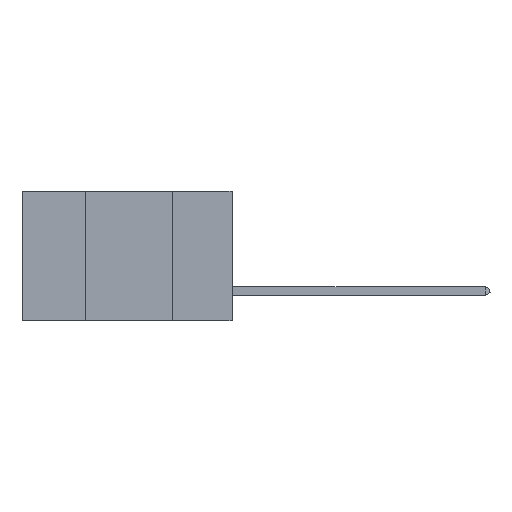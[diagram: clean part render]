
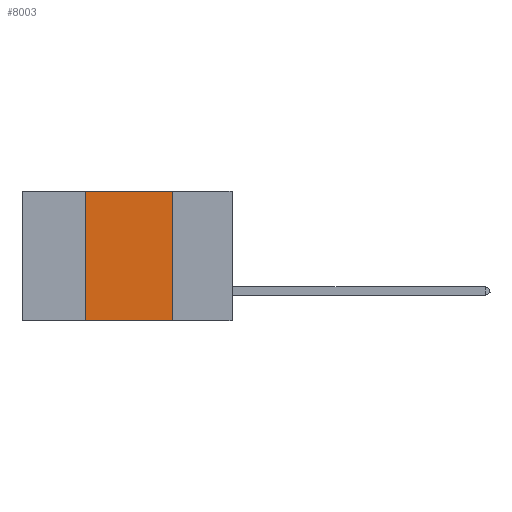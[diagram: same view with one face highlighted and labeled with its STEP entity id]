
A CAD part, left-side view. The second image highlights one B-rep face of the part: STEP entity #8003.
In plain terms, the highlighted planar face has unit normal (-1, 0, 0).
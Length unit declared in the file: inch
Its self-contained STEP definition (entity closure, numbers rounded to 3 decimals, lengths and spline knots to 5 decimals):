
#349 = VERTEX_POINT ( 'NONE', #8921 ) ;
#2960 = CARTESIAN_POINT ( 'NONE',  ( 0., 0.42, 0. ) ) ;
#4209 = VERTEX_POINT ( 'NONE', #22917 ) ;
#7087 = LINE ( 'NONE', #13964, #18270 ) ;
#8003 = ADVANCED_FACE ( 'NONE', ( #25514 ), #35412, .F. ) ;
#8921 = CARTESIAN_POINT ( 'NONE',  ( 0., 0.17, 0. ) ) ;
#9891 = DIRECTION ( 'NONE',  ( 0., -1., 0. ) ) ;
#11871 = VERTEX_POINT ( 'NONE', #13775 ) ;
#12262 = CARTESIAN_POINT ( 'NONE',  ( 0., 0.6, -0.37 ) ) ;
#13615 = VERTEX_POINT ( 'NONE', #2960 ) ;
#13775 = CARTESIAN_POINT ( 'NONE',  ( 0., 0.42, -0.37 ) ) ;
#13964 = CARTESIAN_POINT ( 'NONE',  ( 0., 0.17, 0. ) ) ;
#15202 = DIRECTION ( 'NONE',  ( 1., 0., 0. ) ) ;
#15417 = CARTESIAN_POINT ( 'NONE',  ( 0., 0.6, 0. ) ) ;
#17225 = DIRECTION ( 'NONE',  ( 0., 0., 1. ) ) ;
#18270 = VECTOR ( 'NONE', #40612, 39.37008 ) ;
#18749 = CARTESIAN_POINT ( 'NONE',  ( 0., 0.6, 0. ) ) ;
#19337 = LINE ( 'NONE', #12262, #34757 ) ;
#22237 = EDGE_CURVE ( 'NONE', #11871, #13615, #36586, .T. ) ;
#22614 = EDGE_CURVE ( 'NONE', #349, #4209, #7087, .T. ) ;
#22917 = CARTESIAN_POINT ( 'NONE',  ( 0., 0.17, -0.37 ) ) ;
#23212 = ORIENTED_EDGE ( 'NONE', *, *, #22237, .F. ) ;
#23309 = EDGE_CURVE ( 'NONE', #13615, #349, #34316, .T. ) ;
#25514 = FACE_OUTER_BOUND ( 'NONE', #37423, .T. ) ;
#33944 = AXIS2_PLACEMENT_3D ( 'NONE', #15417, #15202, #38408 ) ;
#34316 = LINE ( 'NONE', #18749, #36861 ) ;
#34451 = ORIENTED_EDGE ( 'NONE', *, *, #23309, .F. ) ;
#34757 = VECTOR ( 'NONE', #9891, 39.37008 ) ;
#35412 = PLANE ( 'NONE',  #33944 ) ;
#35606 = EDGE_CURVE ( 'NONE', #11871, #4209, #19337, .T. ) ;
#36586 = LINE ( 'NONE', #36799, #41613 ) ;
#36799 = CARTESIAN_POINT ( 'NONE',  ( 0., 0.42, 0. ) ) ;
#36861 = VECTOR ( 'NONE', #38534, 39.37008 ) ;
#37037 = ORIENTED_EDGE ( 'NONE', *, *, #35606, .T. ) ;
#37423 = EDGE_LOOP ( 'NONE', ( #37612, #34451, #23212, #37037 ) ) ;
#37612 = ORIENTED_EDGE ( 'NONE', *, *, #22614, .F. ) ;
#38408 = DIRECTION ( 'NONE',  ( 0., 0., -1. ) ) ;
#38534 = DIRECTION ( 'NONE',  ( 0., -1., 0. ) ) ;
#40612 = DIRECTION ( 'NONE',  ( 0., 0., -1. ) ) ;
#41613 = VECTOR ( 'NONE', #17225, 39.37008 ) ;
